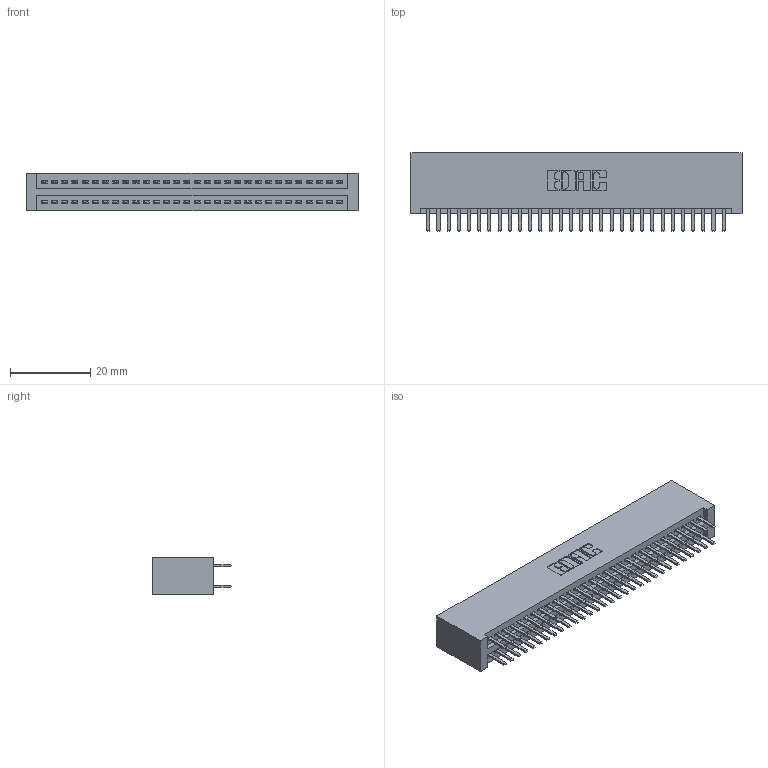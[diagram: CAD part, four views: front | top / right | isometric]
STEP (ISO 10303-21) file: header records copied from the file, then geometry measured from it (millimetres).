
FILE_DESCRIPTION (( 'STEP AP203' ), '1' );
FILE_NAME ('345-060-520-201.STEP', '2019-10-30T07:01:19', ( '' ), ( '' ), 'SwSTEP 2.0', 'SolidWorks 2016', '' );
FILE_SCHEMA (( 'CONFIG_CONTROL_DESIGN' ));
Length unit declared in the file: inch
Products named in the file (3): 345-292-001_345-293-120; 345-060-520-201; 345 Part_No Mounting Lugs
Assembly tree (61 placements, depth 2):
  345-060-520-201
    345 Part_No Mounting Lugs
    345-292-001_345-293-120  x60
Bounding box: 82.8 x 19.68 x 9.4 mm (x, y, z)
Volume: 8521.8 mm3; surface area: 12611.4 mm2
Topology: 61 solids, 61 shells, 3358 faces, 9737 edges, 6330 vertices
Faces by surface type: plane 2176, cylinder 1182
Entity records: 24991 total; most frequent: CARTESIAN_POINT 4212, ORIENTED_EDGE 4134, DIRECTION 3711, EDGE_CURVE 2067, VECTOR 1819, LINE 1819, VERTEX_POINT 1374, AXIS2_PLACEMENT_3D 946
